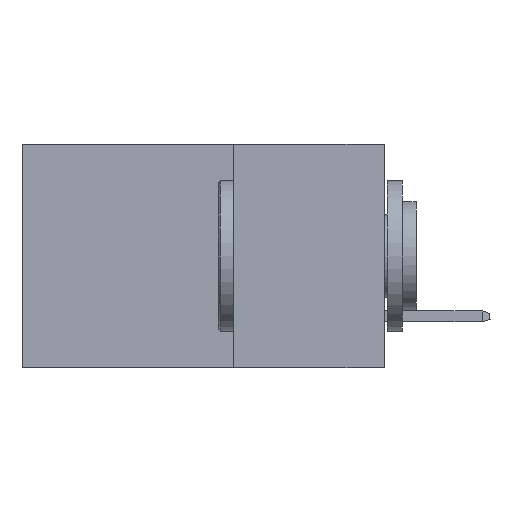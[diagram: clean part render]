
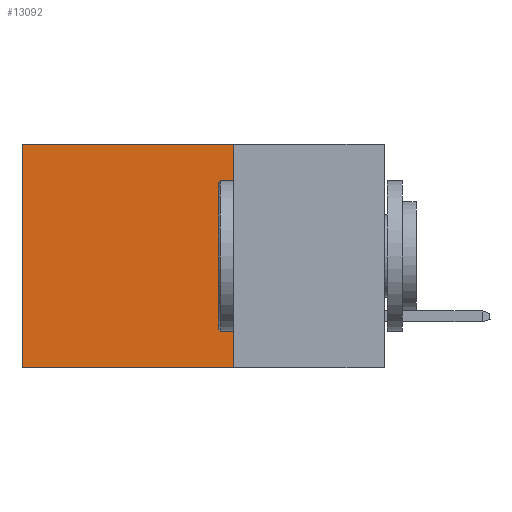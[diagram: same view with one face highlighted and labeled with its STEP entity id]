
A CAD part, left-side view. The second image highlights one B-rep face of the part: STEP entity #13092.
In plain terms, the highlighted planar face has unit normal (-1, 0, 0).
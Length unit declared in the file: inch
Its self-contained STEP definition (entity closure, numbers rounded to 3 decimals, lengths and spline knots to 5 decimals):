
#129 = ORIENTED_EDGE ( 'NONE', *, *, #1773, .T. ) ;
#1773 = EDGE_CURVE ( 'NONE', #13104, #13456, #20850, .T. ) ;
#3017 = ORIENTED_EDGE ( 'NONE', *, *, #20616, .T. ) ;
#3502 = DIRECTION ( 'NONE',  ( 0., 1., 0. ) ) ;
#3679 = CARTESIAN_POINT ( 'NONE',  ( 0.2615, 0.25, -0.37 ) ) ;
#5774 = DIRECTION ( 'NONE',  ( 0., 0., -1. ) ) ;
#7307 = DIRECTION ( 'NONE',  ( 0., 0., -1. ) ) ;
#8732 = FACE_OUTER_BOUND ( 'NONE', #17741, .T. ) ;
#8904 = CARTESIAN_POINT ( 'NONE',  ( 0.2615, 0.6, 0. ) ) ;
#9681 = EDGE_CURVE ( 'NONE', #13104, #21614, #13940, .T. ) ;
#9794 = DIRECTION ( 'NONE',  ( 0., 1., 0. ) ) ;
#10175 = CARTESIAN_POINT ( 'NONE',  ( 0.2615, 0.25, 0. ) ) ;
#10359 = CARTESIAN_POINT ( 'NONE',  ( 0.2615, 0.25, -0.37 ) ) ;
#10498 = LINE ( 'NONE', #19239, #15755 ) ;
#11903 = CARTESIAN_POINT ( 'NONE',  ( 0.2615, 0.25, 0. ) ) ;
#13092 = ADVANCED_FACE ( 'NONE', ( #8732 ), #25513, .F. ) ;
#13104 = VERTEX_POINT ( 'NONE', #11903 ) ;
#13367 = VECTOR ( 'NONE', #3502, 39.37008 ) ;
#13456 = VERTEX_POINT ( 'NONE', #8904 ) ;
#13678 = CARTESIAN_POINT ( 'NONE',  ( 0.2615, 0.25, -0.37 ) ) ;
#13940 = LINE ( 'NONE', #14843, #23723 ) ;
#14843 = CARTESIAN_POINT ( 'NONE',  ( 0.2615, 0.25, -0.37 ) ) ;
#15049 = DIRECTION ( 'NONE',  ( 0., 0., -1. ) ) ;
#15472 = VERTEX_POINT ( 'NONE', #17769 ) ;
#15755 = VECTOR ( 'NONE', #7307, 39.37008 ) ;
#17198 = ORIENTED_EDGE ( 'NONE', *, *, #24621, .F. ) ;
#17741 = EDGE_LOOP ( 'NONE', ( #3017, #17198, #22175, #129 ) ) ;
#17766 = DIRECTION ( 'NONE',  ( 1., 0., 0. ) ) ;
#17769 = CARTESIAN_POINT ( 'NONE',  ( 0.2615, 0.6, -0.37 ) ) ;
#18360 = AXIS2_PLACEMENT_3D ( 'NONE', #3679, #17766, #5774 ) ;
#18601 = LINE ( 'NONE', #13678, #13367 ) ;
#19239 = CARTESIAN_POINT ( 'NONE',  ( 0.2615, 0.6, -0.37 ) ) ;
#20616 = EDGE_CURVE ( 'NONE', #13456, #15472, #10498, .T. ) ;
#20850 = LINE ( 'NONE', #10175, #25351 ) ;
#21614 = VERTEX_POINT ( 'NONE', #10359 ) ;
#22175 = ORIENTED_EDGE ( 'NONE', *, *, #9681, .F. ) ;
#23723 = VECTOR ( 'NONE', #15049, 39.37008 ) ;
#24621 = EDGE_CURVE ( 'NONE', #21614, #15472, #18601, .T. ) ;
#25351 = VECTOR ( 'NONE', #9794, 39.37008 ) ;
#25513 = PLANE ( 'NONE',  #18360 ) ;
